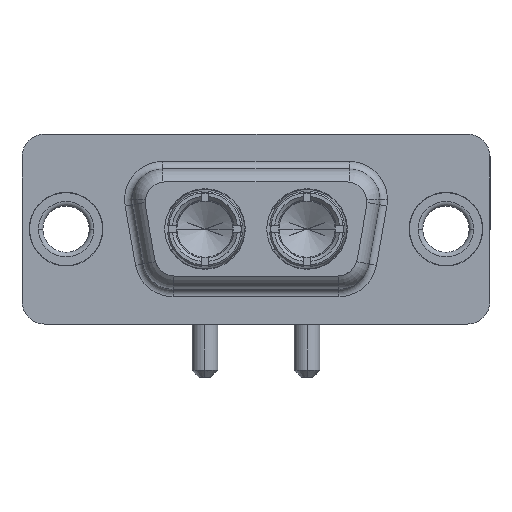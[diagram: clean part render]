
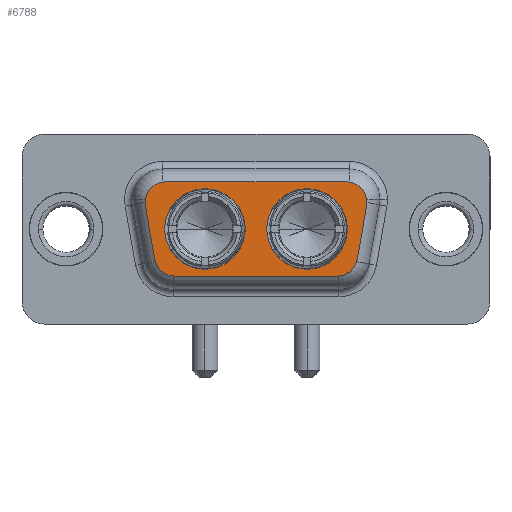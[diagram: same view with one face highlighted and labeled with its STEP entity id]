
A CAD part, top view. The second image highlights one B-rep face of the part: STEP entity #6788.
In plain terms, the highlighted planar face has unit normal (0, 0, 1).
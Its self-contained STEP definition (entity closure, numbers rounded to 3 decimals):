
#11 = DIRECTION ( 'NONE',  ( 0., 0., -1. ) ) ;
#31 = DIRECTION ( 'NONE',  ( 0.174, 0.985, 0. ) ) ;
#75 = VERTEX_POINT ( 'NONE', #101 ) ;
#101 = CARTESIAN_POINT ( 'NONE',  ( 6.55, 3.1, 6.2 ) ) ;
#123 = ORIENTED_EDGE ( 'NONE', *, *, #6661, .T. ) ;
#132 = DIRECTION ( 'NONE',  ( 1., 0., 0. ) ) ;
#390 = EDGE_CURVE ( 'NONE', #6110, #2304, #2693, .T. ) ;
#758 = CARTESIAN_POINT ( 'NONE',  ( 15.86, 0., 6.2 ) ) ;
#916 = EDGE_CURVE ( 'NONE', #6729, #3990, #4548, .T. ) ;
#968 = DIRECTION ( 'NONE',  ( 1., 0., 0. ) ) ;
#1291 = CIRCLE ( 'NONE', #6314, 2.65 ) ;
#1312 = EDGE_LOOP ( 'NONE', ( #8141, #7293 ) ) ;
#1511 = DIRECTION ( 'NONE',  ( 1., 0., 0. ) ) ;
#1588 = FACE_OUTER_BOUND ( 'NONE', #10050, .T. ) ;
#1662 = CIRCLE ( 'NONE', #8537, 1.35 ) ;
#1727 = EDGE_CURVE ( 'NONE', #3990, #6110, #10380, .T. ) ;
#1814 = DIRECTION ( 'NONE',  ( 0., 0., 1. ) ) ;
#1988 = CARTESIAN_POINT ( 'NONE',  ( 5.221, 1.516, 6.2 ) ) ;
#2010 = DIRECTION ( 'NONE',  ( 0.174, -0.985, 0. ) ) ;
#2304 = VERTEX_POINT ( 'NONE', #9876 ) ;
#2340 = CARTESIAN_POINT ( 'NONE',  ( 17.833, -3.1, 6.2 ) ) ;
#2487 = DIRECTION ( 'NONE',  ( 1., 0., 0. ) ) ;
#2509 = CARTESIAN_POINT ( 'NONE',  ( 5.2, 1.75, 6.2 ) ) ;
#2693 = CIRCLE ( 'NONE', #9083, 1.35 ) ;
#2784 = DIRECTION ( 'NONE',  ( 1., 0., 0. ) ) ;
#2786 = VERTEX_POINT ( 'NONE', #1988 ) ;
#2886 = VECTOR ( 'NONE', #2010, 1000. ) ;
#2978 = EDGE_LOOP ( 'NONE', ( #8781, #9550 ) ) ;
#3064 = CARTESIAN_POINT ( 'NONE',  ( 9.14, 0., 6.2 ) ) ;
#3172 = EDGE_CURVE ( 'NONE', #5573, #5140, #8944, .T. ) ;
#3199 = CARTESIAN_POINT ( 'NONE',  ( 11.79, 0., 6.2 ) ) ;
#3362 = DIRECTION ( 'NONE',  ( 0., 0., 1. ) ) ;
#3380 = EDGE_CURVE ( 'NONE', #5250, #9386, #6086, .T. ) ;
#3423 = CIRCLE ( 'NONE', #4945, 2.65 ) ;
#3479 = DIRECTION ( 'NONE',  ( 1., 0., 0. ) ) ;
#3584 = EDGE_CURVE ( 'NONE', #6917, #2786, #9289, .T. ) ;
#3719 = AXIS2_PLACEMENT_3D ( 'NONE', #5119, #7435, #3479 ) ;
#3720 = CARTESIAN_POINT ( 'NONE',  ( 5.838, -1.984, 6.2 ) ) ;
#3728 = AXIS2_PLACEMENT_3D ( 'NONE', #3064, #7901, #4591 ) ;
#3763 = CARTESIAN_POINT ( 'NONE',  ( 18.45, 1.75, 6.2 ) ) ;
#3977 = ORIENTED_EDGE ( 'NONE', *, *, #6218, .T. ) ;
#3985 = CARTESIAN_POINT ( 'NONE',  ( 7.167, -3.1, 6.2 ) ) ;
#3990 = VERTEX_POINT ( 'NONE', #3985 ) ;
#4361 = LINE ( 'NONE', #7574, #2886 ) ;
#4400 = DIRECTION ( 'NONE',  ( -1., 0., 0. ) ) ;
#4531 = CARTESIAN_POINT ( 'NONE',  ( 13.21, 0., 6.2 ) ) ;
#4548 = CIRCLE ( 'NONE', #6058, 1.35 ) ;
#4591 = DIRECTION ( 'NONE',  ( 1., 0., 0. ) ) ;
#4597 = DIRECTION ( 'NONE',  ( -1., 0., 0. ) ) ;
#4667 = CARTESIAN_POINT ( 'NONE',  ( 19.779, 1.516, 6.2 ) ) ;
#4670 = ORIENTED_EDGE ( 'NONE', *, *, #7070, .T. ) ;
#4681 = CARTESIAN_POINT ( 'NONE',  ( 7.167, -1.75, 6.2 ) ) ;
#4751 = ORIENTED_EDGE ( 'NONE', *, *, #390, .T. ) ;
#4784 = EDGE_CURVE ( 'NONE', #5140, #5573, #1291, .T. ) ;
#4795 = VECTOR ( 'NONE', #31, 1000. ) ;
#4899 = CARTESIAN_POINT ( 'NONE',  ( 17.833, -3.1, 6.2 ) ) ;
#4910 = VERTEX_POINT ( 'NONE', #10377 ) ;
#4945 = AXIS2_PLACEMENT_3D ( 'NONE', #10274, #7020, #1511 ) ;
#4949 = DIRECTION ( 'NONE',  ( 0., 0., 1. ) ) ;
#5068 = AXIS2_PLACEMENT_3D ( 'NONE', #9838, #1814, #132 ) ;
#5119 = CARTESIAN_POINT ( 'NONE',  ( 15.86, 0., 6.2 ) ) ;
#5140 = VERTEX_POINT ( 'NONE', #4531 ) ;
#5228 = CIRCLE ( 'NONE', #5068, 1.35 ) ;
#5250 = VERTEX_POINT ( 'NONE', #7790 ) ;
#5448 = LINE ( 'NONE', #4667, #4795 ) ;
#5564 = DIRECTION ( 'NONE',  ( -1., 0., 0. ) ) ;
#5573 = VERTEX_POINT ( 'NONE', #7831 ) ;
#5649 = ORIENTED_EDGE ( 'NONE', *, *, #5654, .T. ) ;
#5654 = EDGE_CURVE ( 'NONE', #9704, #4910, #1662, .T. ) ;
#5973 = CARTESIAN_POINT ( 'NONE',  ( 19.779, 1.516, 6.2 ) ) ;
#6020 = CARTESIAN_POINT ( 'NONE',  ( 6.55, 3.1, 6.2 ) ) ;
#6058 = AXIS2_PLACEMENT_3D ( 'NONE', #4681, #10356, #6295 ) ;
#6086 = CIRCLE ( 'NONE', #3728, 2.65 ) ;
#6110 = VERTEX_POINT ( 'NONE', #4899 ) ;
#6146 = VECTOR ( 'NONE', #4400, 1000. ) ;
#6186 = DIRECTION ( 'NONE',  ( 0., 0., 1. ) ) ;
#6218 = EDGE_CURVE ( 'NONE', #2304, #9704, #5448, .T. ) ;
#6295 = DIRECTION ( 'NONE',  ( -1., 0., 0. ) ) ;
#6314 = AXIS2_PLACEMENT_3D ( 'NONE', #758, #4949, #968 ) ;
#6398 = PLANE ( 'NONE',  #7277 ) ;
#6661 = EDGE_CURVE ( 'NONE', #2786, #6729, #4361, .T. ) ;
#6729 = VERTEX_POINT ( 'NONE', #3720 ) ;
#6788 = ADVANCED_FACE ( 'NONE', ( #7201, #7887, #1588 ), #6398, .F. ) ;
#6860 = ORIENTED_EDGE ( 'NONE', *, *, #3584, .T. ) ;
#6912 = ORIENTED_EDGE ( 'NONE', *, *, #1727, .T. ) ;
#6917 = VERTEX_POINT ( 'NONE', #2509 ) ;
#7020 = DIRECTION ( 'NONE',  ( 0., 0., 1. ) ) ;
#7070 = EDGE_CURVE ( 'NONE', #4910, #75, #9241, .T. ) ;
#7201 = FACE_BOUND ( 'NONE', #2978, .T. ) ;
#7277 = AXIS2_PLACEMENT_3D ( 'NONE', #7993, #11, #5564 ) ;
#7293 = ORIENTED_EDGE ( 'NONE', *, *, #3380, .F. ) ;
#7435 = DIRECTION ( 'NONE',  ( 0., 0., 1. ) ) ;
#7574 = CARTESIAN_POINT ( 'NONE',  ( 5.838, -1.984, 6.2 ) ) ;
#7597 = CARTESIAN_POINT ( 'NONE',  ( 17.833, -1.75, 6.2 ) ) ;
#7733 = VECTOR ( 'NONE', #2487, 1000. ) ;
#7787 = EDGE_CURVE ( 'NONE', #75, #6917, #5228, .T. ) ;
#7790 = CARTESIAN_POINT ( 'NONE',  ( 6.49, 0., 6.2 ) ) ;
#7831 = CARTESIAN_POINT ( 'NONE',  ( 18.51, 0., 6.2 ) ) ;
#7887 = FACE_BOUND ( 'NONE', #1312, .T. ) ;
#7901 = DIRECTION ( 'NONE',  ( 0., 0., 1. ) ) ;
#7993 = CARTESIAN_POINT ( 'NONE',  ( 7.167, -1.75, 6.2 ) ) ;
#8141 = ORIENTED_EDGE ( 'NONE', *, *, #9062, .F. ) ;
#8279 = AXIS2_PLACEMENT_3D ( 'NONE', #9984, #3362, #2784 ) ;
#8423 = ORIENTED_EDGE ( 'NONE', *, *, #916, .T. ) ;
#8537 = AXIS2_PLACEMENT_3D ( 'NONE', #3763, #6186, #9358 ) ;
#8600 = DIRECTION ( 'NONE',  ( 0., 0., 1. ) ) ;
#8781 = ORIENTED_EDGE ( 'NONE', *, *, #3172, .F. ) ;
#8944 = CIRCLE ( 'NONE', #3719, 2.65 ) ;
#9012 = ORIENTED_EDGE ( 'NONE', *, *, #7787, .T. ) ;
#9062 = EDGE_CURVE ( 'NONE', #9386, #5250, #3423, .T. ) ;
#9083 = AXIS2_PLACEMENT_3D ( 'NONE', #7597, #8600, #4597 ) ;
#9241 = LINE ( 'NONE', #6020, #6146 ) ;
#9289 = CIRCLE ( 'NONE', #8279, 1.35 ) ;
#9358 = DIRECTION ( 'NONE',  ( -1., 0., 0. ) ) ;
#9386 = VERTEX_POINT ( 'NONE', #3199 ) ;
#9550 = ORIENTED_EDGE ( 'NONE', *, *, #4784, .F. ) ;
#9704 = VERTEX_POINT ( 'NONE', #5973 ) ;
#9838 = CARTESIAN_POINT ( 'NONE',  ( 6.55, 1.75, 6.2 ) ) ;
#9876 = CARTESIAN_POINT ( 'NONE',  ( 19.162, -1.984, 6.2 ) ) ;
#9984 = CARTESIAN_POINT ( 'NONE',  ( 6.55, 1.75, 6.2 ) ) ;
#10050 = EDGE_LOOP ( 'NONE', ( #8423, #6912, #4751, #3977, #5649, #4670, #9012, #6860, #123 ) ) ;
#10274 = CARTESIAN_POINT ( 'NONE',  ( 9.14, 0., 6.2 ) ) ;
#10356 = DIRECTION ( 'NONE',  ( 0., 0., 1. ) ) ;
#10377 = CARTESIAN_POINT ( 'NONE',  ( 18.45, 3.1, 6.2 ) ) ;
#10380 = LINE ( 'NONE', #2340, #7733 ) ;
